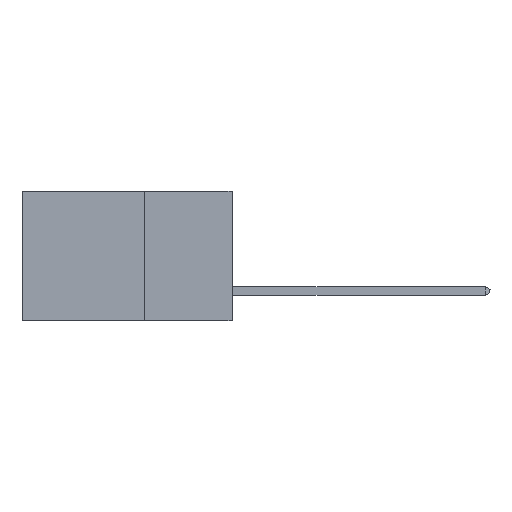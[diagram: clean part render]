
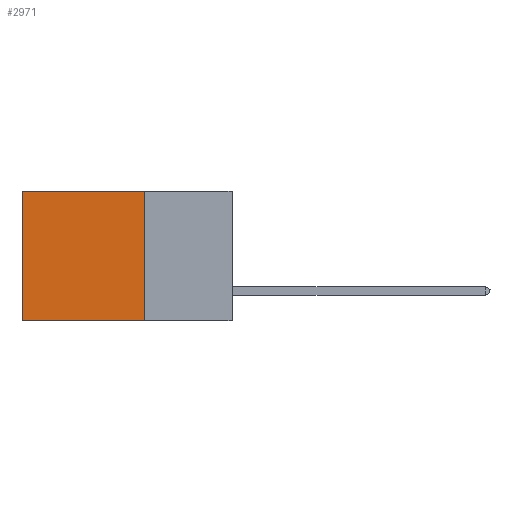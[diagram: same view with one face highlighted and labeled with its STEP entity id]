
A CAD part, left-side view. The second image highlights one B-rep face of the part: STEP entity #2971.
In plain terms, the highlighted planar face has unit normal (-1, 0, 0).
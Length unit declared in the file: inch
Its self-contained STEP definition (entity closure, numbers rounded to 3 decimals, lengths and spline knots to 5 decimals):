
#1883 = AXIS2_PLACEMENT_3D ( 'NONE', #27339, #24228, #9107 ) ;
#2971 = ADVANCED_FACE ( 'NONE', ( #3418 ), #20820, .F. ) ;
#3418 = FACE_OUTER_BOUND ( 'NONE', #15454, .T. ) ;
#3635 = VERTEX_POINT ( 'NONE', #10210 ) ;
#4922 = CARTESIAN_POINT ( 'NONE',  ( 0.2875, 0.25, -0.37 ) ) ;
#5554 = ORIENTED_EDGE ( 'NONE', *, *, #18229, .F. ) ;
#6030 = CARTESIAN_POINT ( 'NONE',  ( 0.2875, 0.25, 0. ) ) ;
#7772 = VECTOR ( 'NONE', #38261, 39.37008 ) ;
#9107 = DIRECTION ( 'NONE',  ( 0., 0., -1. ) ) ;
#9597 = EDGE_CURVE ( 'NONE', #28242, #22907, #31068, .T. ) ;
#10091 = LINE ( 'NONE', #32344, #29695 ) ;
#10210 = CARTESIAN_POINT ( 'NONE',  ( 0.2875, 0.25, 0. ) ) ;
#12464 = LINE ( 'NONE', #6030, #23404 ) ;
#12510 = EDGE_CURVE ( 'NONE', #17044, #22907, #27837, .T. ) ;
#12945 = CARTESIAN_POINT ( 'NONE',  ( 0.2875, 0.25, -0.37 ) ) ;
#13056 = CARTESIAN_POINT ( 'NONE',  ( 0.2875, 0.6, 0. ) ) ;
#13111 = ORIENTED_EDGE ( 'NONE', *, *, #23341, .T. ) ;
#14961 = VECTOR ( 'NONE', #37112, 39.37008 ) ;
#15089 = CARTESIAN_POINT ( 'NONE',  ( 0.2875, 0.6, 0. ) ) ;
#15454 = EDGE_LOOP ( 'NONE', ( #19778, #28574, #5554, #13111 ) ) ;
#17044 = VERTEX_POINT ( 'NONE', #15089 ) ;
#18229 = EDGE_CURVE ( 'NONE', #3635, #28242, #10091, .T. ) ;
#19778 = ORIENTED_EDGE ( 'NONE', *, *, #12510, .T. ) ;
#20820 = PLANE ( 'NONE',  #1883 ) ;
#21655 = DIRECTION ( 'NONE',  ( 0., 1., 0. ) ) ;
#22907 = VERTEX_POINT ( 'NONE', #30622 ) ;
#23341 = EDGE_CURVE ( 'NONE', #3635, #17044, #12464, .T. ) ;
#23404 = VECTOR ( 'NONE', #21655, 39.37008 ) ;
#24228 = DIRECTION ( 'NONE',  ( 1., 0., 0. ) ) ;
#27339 = CARTESIAN_POINT ( 'NONE',  ( 0.2875, 0.25, 0. ) ) ;
#27837 = LINE ( 'NONE', #13056, #7772 ) ;
#28242 = VERTEX_POINT ( 'NONE', #12945 ) ;
#28574 = ORIENTED_EDGE ( 'NONE', *, *, #9597, .F. ) ;
#29695 = VECTOR ( 'NONE', #35399, 39.37008 ) ;
#30622 = CARTESIAN_POINT ( 'NONE',  ( 0.2875, 0.6, -0.37 ) ) ;
#31068 = LINE ( 'NONE', #4922, #14961 ) ;
#32344 = CARTESIAN_POINT ( 'NONE',  ( 0.2875, 0.25, 0. ) ) ;
#35399 = DIRECTION ( 'NONE',  ( 0., 0., -1. ) ) ;
#37112 = DIRECTION ( 'NONE',  ( 0., 1., 0. ) ) ;
#38261 = DIRECTION ( 'NONE',  ( 0., 0., -1. ) ) ;
